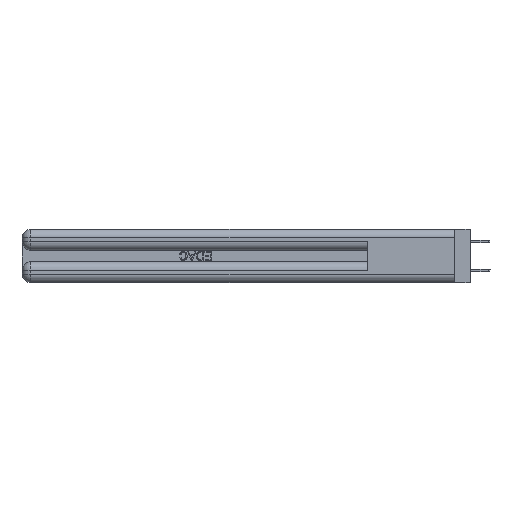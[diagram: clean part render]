
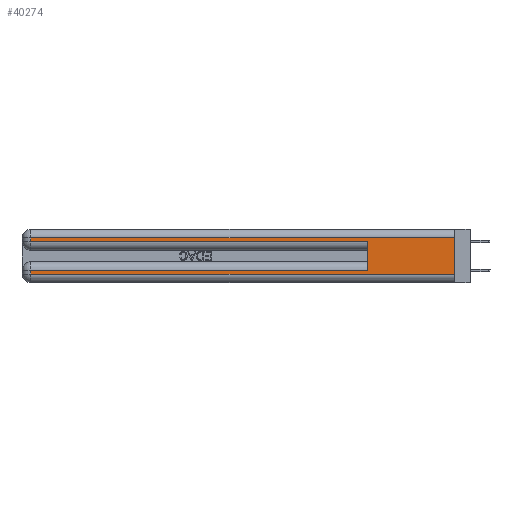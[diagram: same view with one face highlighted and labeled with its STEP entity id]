
A CAD part, left-side view. The second image highlights one B-rep face of the part: STEP entity #40274.
In plain terms, the highlighted planar face has unit normal (-1, 0, 0).
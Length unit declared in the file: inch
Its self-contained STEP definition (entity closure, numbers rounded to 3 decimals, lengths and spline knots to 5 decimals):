
#659 = LINE ( 'NONE', #29632, #6690 ) ;
#1814 = VERTEX_POINT ( 'NONE', #33179 ) ;
#2951 = DIRECTION ( 'NONE',  ( 0., 1., 0. ) ) ;
#3448 = EDGE_CURVE ( 'NONE', #39337, #12982, #659, .T. ) ;
#4359 = EDGE_CURVE ( 'NONE', #13115, #25224, #33481, .T. ) ;
#4736 = LINE ( 'NONE', #15465, #9357 ) ;
#5176 = VECTOR ( 'NONE', #22328, 39.37008 ) ;
#6690 = VECTOR ( 'NONE', #14929, 39.37008 ) ;
#6869 = CARTESIAN_POINT ( 'NONE',  ( 0., 0., 0.37 ) ) ;
#8246 = DIRECTION ( 'NONE',  ( 0., 0., -1. ) ) ;
#8603 = CARTESIAN_POINT ( 'NONE',  ( 0., 0., 0.285 ) ) ;
#8743 = ORIENTED_EDGE ( 'NONE', *, *, #11478, .T. ) ;
#9357 = VECTOR ( 'NONE', #39769, 39.37008 ) ;
#10056 = CARTESIAN_POINT ( 'NONE',  ( 0., 2.94, 0.37 ) ) ;
#10075 = CARTESIAN_POINT ( 'NONE',  ( 0., 2.94, 0.06 ) ) ;
#10122 = PLANE ( 'NONE',  #36053 ) ;
#10576 = DIRECTION ( 'NONE',  ( 0., 0., -1. ) ) ;
#11478 = EDGE_CURVE ( 'NONE', #18040, #12982, #15153, .T. ) ;
#12058 = CARTESIAN_POINT ( 'NONE',  ( 0., 2.94, 0.085 ) ) ;
#12269 = EDGE_CURVE ( 'NONE', #25224, #1814, #22754, .T. ) ;
#12982 = VERTEX_POINT ( 'NONE', #32293 ) ;
#13115 = VERTEX_POINT ( 'NONE', #12058 ) ;
#13559 = EDGE_LOOP ( 'NONE', ( #45421, #44534, #25802, #8743, #40369, #16263, #21582, #30697 ) ) ;
#13969 = VECTOR ( 'NONE', #22641, 39.37008 ) ;
#14809 = CARTESIAN_POINT ( 'NONE',  ( 0., 0., 0.06 ) ) ;
#14929 = DIRECTION ( 'NONE',  ( 0., 0., 1. ) ) ;
#15045 = EDGE_CURVE ( 'NONE', #37662, #18040, #26458, .T. ) ;
#15153 = LINE ( 'NONE', #8603, #13969 ) ;
#15465 = CARTESIAN_POINT ( 'NONE',  ( 0., 0., 0.37 ) ) ;
#16263 = ORIENTED_EDGE ( 'NONE', *, *, #20149, .T. ) ;
#17672 = CARTESIAN_POINT ( 'NONE',  ( 0., 0., 0.085 ) ) ;
#18040 = VERTEX_POINT ( 'NONE', #38118 ) ;
#20149 = EDGE_CURVE ( 'NONE', #39337, #13115, #35649, .T. ) ;
#21582 = ORIENTED_EDGE ( 'NONE', *, *, #4359, .T. ) ;
#21823 = CARTESIAN_POINT ( 'NONE',  ( 0., 0., 0.31 ) ) ;
#22095 = CARTESIAN_POINT ( 'NONE',  ( 0., 0., 0.31 ) ) ;
#22328 = DIRECTION ( 'NONE',  ( 0., 1., 0. ) ) ;
#22641 = DIRECTION ( 'NONE',  ( 0., -1., 0. ) ) ;
#22754 = LINE ( 'NONE', #14809, #39618 ) ;
#22757 = DIRECTION ( 'NONE',  ( 0., 0., -1. ) ) ;
#25053 = VECTOR ( 'NONE', #22757, 39.37008 ) ;
#25224 = VERTEX_POINT ( 'NONE', #10075 ) ;
#25802 = ORIENTED_EDGE ( 'NONE', *, *, #15045, .T. ) ;
#26458 = LINE ( 'NONE', #40917, #28831 ) ;
#28831 = VECTOR ( 'NONE', #8246, 39.37008 ) ;
#29133 = VERTEX_POINT ( 'NONE', #21823 ) ;
#29214 = EDGE_CURVE ( 'NONE', #29133, #1814, #4736, .T. ) ;
#29474 = CARTESIAN_POINT ( 'NONE',  ( 0., 0.6, 0.085 ) ) ;
#29632 = CARTESIAN_POINT ( 'NONE',  ( 0., 0.6, 0.145 ) ) ;
#30697 = ORIENTED_EDGE ( 'NONE', *, *, #12269, .T. ) ;
#30925 = CARTESIAN_POINT ( 'NONE',  ( 0., 2.94, 0.31 ) ) ;
#32293 = CARTESIAN_POINT ( 'NONE',  ( 0., 0.6, 0.285 ) ) ;
#33179 = CARTESIAN_POINT ( 'NONE',  ( 0., 0., 0.06 ) ) ;
#33481 = LINE ( 'NONE', #10056, #25053 ) ;
#33598 = EDGE_CURVE ( 'NONE', #29133, #37662, #43562, .T. ) ;
#34888 = FACE_OUTER_BOUND ( 'NONE', #13559, .T. ) ;
#35649 = LINE ( 'NONE', #17672, #41758 ) ;
#36053 = AXIS2_PLACEMENT_3D ( 'NONE', #6869, #42345, #10576 ) ;
#37662 = VERTEX_POINT ( 'NONE', #30925 ) ;
#38118 = CARTESIAN_POINT ( 'NONE',  ( 0., 2.94, 0.285 ) ) ;
#39337 = VERTEX_POINT ( 'NONE', #29474 ) ;
#39618 = VECTOR ( 'NONE', #40477, 39.37008 ) ;
#39769 = DIRECTION ( 'NONE',  ( 0., 0., -1. ) ) ;
#40274 = ADVANCED_FACE ( 'NONE', ( #34888 ), #10122, .F. ) ;
#40369 = ORIENTED_EDGE ( 'NONE', *, *, #3448, .F. ) ;
#40477 = DIRECTION ( 'NONE',  ( 0., -1., 0. ) ) ;
#40917 = CARTESIAN_POINT ( 'NONE',  ( 0., 2.94, 0.37 ) ) ;
#41758 = VECTOR ( 'NONE', #2951, 39.37008 ) ;
#42345 = DIRECTION ( 'NONE',  ( 1., 0., 0. ) ) ;
#43562 = LINE ( 'NONE', #22095, #5176 ) ;
#44534 = ORIENTED_EDGE ( 'NONE', *, *, #33598, .T. ) ;
#45421 = ORIENTED_EDGE ( 'NONE', *, *, #29214, .F. ) ;
